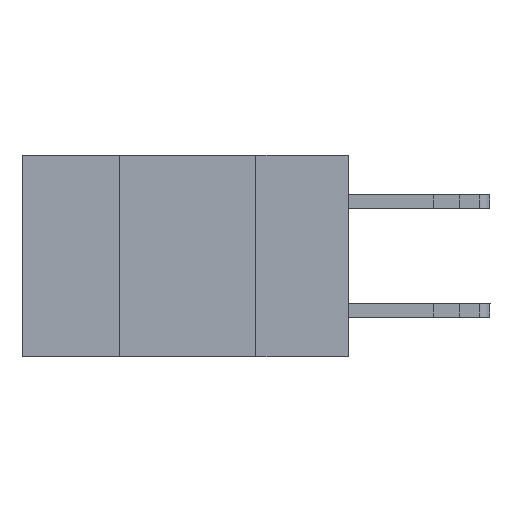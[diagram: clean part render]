
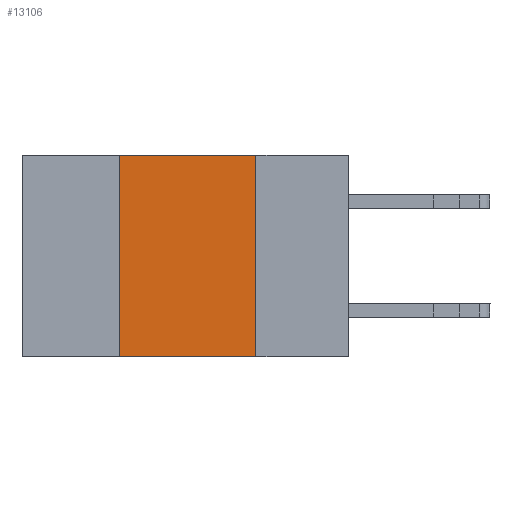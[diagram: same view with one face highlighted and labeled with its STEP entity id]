
A CAD part, left-side view. The second image highlights one B-rep face of the part: STEP entity #13106.
In plain terms, the highlighted planar face has unit normal (-1, 0, 0).
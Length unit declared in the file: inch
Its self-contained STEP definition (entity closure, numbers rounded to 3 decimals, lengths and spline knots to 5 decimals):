
#659 = VECTOR ( 'NONE', #3363, 39.37008 ) ;
#1101 = CARTESIAN_POINT ( 'NONE',  ( 0., 0.6, 0. ) ) ;
#1660 = CARTESIAN_POINT ( 'NONE',  ( 0., 0.17, 0. ) ) ;
#1680 = ORIENTED_EDGE ( 'NONE', *, *, #7463, .T. ) ;
#2027 = CARTESIAN_POINT ( 'NONE',  ( 0., 0.17, -0.37 ) ) ;
#2269 = VECTOR ( 'NONE', #9792, 39.37008 ) ;
#2541 = DIRECTION ( 'NONE',  ( 0., 0., -1. ) ) ;
#2747 = DIRECTION ( 'NONE',  ( 0., -1., 0. ) ) ;
#2771 = LINE ( 'NONE', #11050, #2269 ) ;
#2964 = LINE ( 'NONE', #12399, #13379 ) ;
#3363 = DIRECTION ( 'NONE',  ( 0., -1., 0. ) ) ;
#3715 = LINE ( 'NONE', #11015, #659 ) ;
#3965 = EDGE_CURVE ( 'NONE', #10274, #11459, #7164, .T. ) ;
#4151 = EDGE_CURVE ( 'NONE', #11459, #9007, #2964, .T. ) ;
#4259 = ORIENTED_EDGE ( 'NONE', *, *, #4151, .F. ) ;
#4976 = EDGE_CURVE ( 'NONE', #10548, #10274, #2771, .T. ) ;
#5392 = PLANE ( 'NONE',  #8102 ) ;
#5475 = DIRECTION ( 'NONE',  ( 0., 0., -1. ) ) ;
#5894 = CARTESIAN_POINT ( 'NONE',  ( 0., 0.6, 0. ) ) ;
#7164 = LINE ( 'NONE', #5894, #13698 ) ;
#7463 = EDGE_CURVE ( 'NONE', #10548, #9007, #3715, .T. ) ;
#8072 = CARTESIAN_POINT ( 'NONE',  ( 0., 0.42, 0. ) ) ;
#8102 = AXIS2_PLACEMENT_3D ( 'NONE', #1101, #10843, #5475 ) ;
#8223 = ORIENTED_EDGE ( 'NONE', *, *, #4976, .F. ) ;
#8371 = EDGE_LOOP ( 'NONE', ( #4259, #12806, #8223, #1680 ) ) ;
#9007 = VERTEX_POINT ( 'NONE', #2027 ) ;
#9792 = DIRECTION ( 'NONE',  ( 0., 0., 1. ) ) ;
#10274 = VERTEX_POINT ( 'NONE', #8072 ) ;
#10548 = VERTEX_POINT ( 'NONE', #12290 ) ;
#10843 = DIRECTION ( 'NONE',  ( 1., 0., 0. ) ) ;
#11015 = CARTESIAN_POINT ( 'NONE',  ( 0., 0.6, -0.37 ) ) ;
#11050 = CARTESIAN_POINT ( 'NONE',  ( 0., 0.42, 0. ) ) ;
#11252 = FACE_OUTER_BOUND ( 'NONE', #8371, .T. ) ;
#11459 = VERTEX_POINT ( 'NONE', #1660 ) ;
#12290 = CARTESIAN_POINT ( 'NONE',  ( 0., 0.42, -0.37 ) ) ;
#12399 = CARTESIAN_POINT ( 'NONE',  ( 0., 0.17, 0. ) ) ;
#12806 = ORIENTED_EDGE ( 'NONE', *, *, #3965, .F. ) ;
#13106 = ADVANCED_FACE ( 'NONE', ( #11252 ), #5392, .F. ) ;
#13379 = VECTOR ( 'NONE', #2541, 39.37008 ) ;
#13698 = VECTOR ( 'NONE', #2747, 39.37008 ) ;
